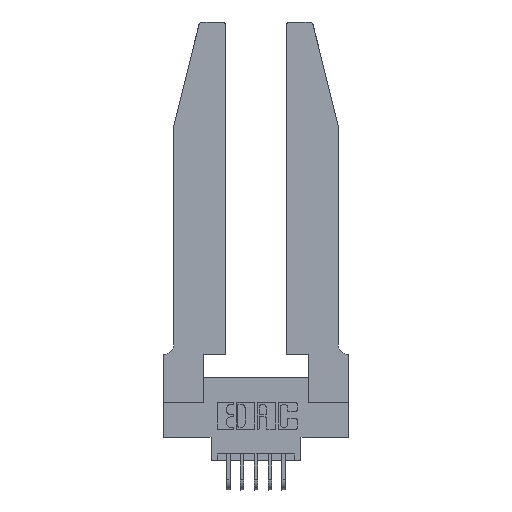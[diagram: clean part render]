
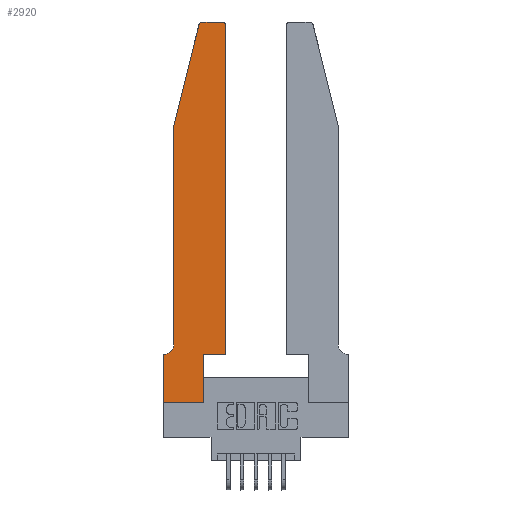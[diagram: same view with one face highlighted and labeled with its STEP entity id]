
A CAD part, top view. The second image highlights one B-rep face of the part: STEP entity #2920.
In plain terms, the highlighted planar face has unit normal (0, 0, 1).
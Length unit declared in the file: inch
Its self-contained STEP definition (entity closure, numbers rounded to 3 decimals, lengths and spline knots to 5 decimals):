
#267 = DIRECTION ( 'NONE',  ( 0., -1., 0. ) ) ;
#280 = EDGE_CURVE ( 'NONE', #4974, #8534, #6755, .T. ) ;
#390 = LINE ( 'NONE', #2423, #12693 ) ;
#575 = CARTESIAN_POINT ( 'NONE',  ( 0.4205, 2.72, 0.37 ) ) ;
#576 = DIRECTION ( 'NONE',  ( 1., 0., 0. ) ) ;
#625 = DIRECTION ( 'NONE',  ( 1., 0., 0. ) ) ;
#717 = VECTOR ( 'NONE', #1704, 39.37008 ) ;
#777 = DIRECTION ( 'NONE',  ( 1., 0., 0. ) ) ;
#1067 = ORIENTED_EDGE ( 'NONE', *, *, #4569, .T. ) ;
#1070 = VERTEX_POINT ( 'NONE', #10532 ) ;
#1077 = EDGE_CURVE ( 'NONE', #4889, #1070, #390, .T. ) ;
#1092 = VECTOR ( 'NONE', #5197, 39.37008 ) ;
#1368 = VECTOR ( 'NONE', #12959, 39.37008 ) ;
#1704 = DIRECTION ( 'NONE',  ( 0., 1., 0. ) ) ;
#1723 = CARTESIAN_POINT ( 'NONE',  ( 0.2865, 0.35, 0.37 ) ) ;
#1918 = DIRECTION ( 'NONE',  ( 0., 0., 1. ) ) ;
#2266 = CARTESIAN_POINT ( 'NONE',  ( 0.4505, 0.35, 0.37 ) ) ;
#2324 = ORIENTED_EDGE ( 'NONE', *, *, #12569, .T. ) ;
#2423 = CARTESIAN_POINT ( 'NONE',  ( 0.0755, 2., 0.37 ) ) ;
#2869 = CARTESIAN_POINT ( 'NONE',  ( 0.2865, 0.35, 0.37 ) ) ;
#2920 = ADVANCED_FACE ( 'NONE', ( #13415 ), #8913, .T. ) ;
#2939 = CARTESIAN_POINT ( 'NONE',  ( 0., 0.35, 0.37 ) ) ;
#2942 = VERTEX_POINT ( 'NONE', #2939 ) ;
#2949 = VERTEX_POINT ( 'NONE', #1723 ) ;
#3039 = DIRECTION ( 'NONE',  ( -1., 0., 0. ) ) ;
#3297 = CARTESIAN_POINT ( 'NONE',  ( 0.284, 2.72, 0.37 ) ) ;
#3588 = VERTEX_POINT ( 'NONE', #6437 ) ;
#3754 = LINE ( 'NONE', #11415, #14758 ) ;
#3841 = EDGE_LOOP ( 'NONE', ( #4428, #14065, #12921, #6975, #9036, #13709, #1067, #14324, #2324, #7661, #10446, #6878 ) ) ;
#4404 = LINE ( 'NONE', #13679, #4600 ) ;
#4428 = ORIENTED_EDGE ( 'NONE', *, *, #12655, .T. ) ;
#4569 = EDGE_CURVE ( 'NONE', #2942, #5217, #13560, .T. ) ;
#4600 = VECTOR ( 'NONE', #576, 39.37008 ) ;
#4889 = VERTEX_POINT ( 'NONE', #7549 ) ;
#4959 = DIRECTION ( 'NONE',  ( -0.239, -0.971, 0. ) ) ;
#4974 = VERTEX_POINT ( 'NONE', #13524 ) ;
#5197 = DIRECTION ( 'NONE',  ( 0., 1., 0. ) ) ;
#5217 = VERTEX_POINT ( 'NONE', #7340 ) ;
#5251 = CARTESIAN_POINT ( 'NONE',  ( 0.2865, 0., 0.37 ) ) ;
#5362 = CARTESIAN_POINT ( 'NONE',  ( 0.0055, 0.42, 0.37 ) ) ;
#5468 = DIRECTION ( 'NONE',  ( 0., 0., -1. ) ) ;
#5637 = CARTESIAN_POINT ( 'NONE',  ( 0.4505, 0.35, 0.37 ) ) ;
#5806 = DIRECTION ( 'NONE',  ( 0., -1., 0. ) ) ;
#5923 = EDGE_CURVE ( 'NONE', #2949, #13540, #8840, .T. ) ;
#6043 = CIRCLE ( 'NONE', #10051, 0.07 ) ;
#6257 = CARTESIAN_POINT ( 'NONE',  ( 0.0755, 2., 0.37 ) ) ;
#6437 = CARTESIAN_POINT ( 'NONE',  ( 0.4505, 2.72, 0.37 ) ) ;
#6447 = DIRECTION ( 'NONE',  ( -1., 0., 0. ) ) ;
#6755 = CIRCLE ( 'NONE', #14008, 0.03 ) ;
#6868 = LINE ( 'NONE', #11218, #1092 ) ;
#6878 = ORIENTED_EDGE ( 'NONE', *, *, #10476, .T. ) ;
#6975 = ORIENTED_EDGE ( 'NONE', *, *, #1077, .T. ) ;
#7340 = CARTESIAN_POINT ( 'NONE',  ( 0., 0., 0.37 ) ) ;
#7549 = CARTESIAN_POINT ( 'NONE',  ( 0.0755, 2., 0.37 ) ) ;
#7602 = VECTOR ( 'NONE', #267, 39.37008 ) ;
#7613 = EDGE_CURVE ( 'NONE', #11349, #2942, #8636, .T. ) ;
#7642 = CARTESIAN_POINT ( 'NONE',  ( 0., 0.35, 0.37 ) ) ;
#7661 = ORIENTED_EDGE ( 'NONE', *, *, #5923, .T. ) ;
#7710 = AXIS2_PLACEMENT_3D ( 'NONE', #575, #1918, #625 ) ;
#8254 = VECTOR ( 'NONE', #6447, 39.37008 ) ;
#8469 = AXIS2_PLACEMENT_3D ( 'NONE', #7642, #14876, #8807 ) ;
#8534 = VERTEX_POINT ( 'NONE', #14683 ) ;
#8636 = LINE ( 'NONE', #13449, #8254 ) ;
#8807 = DIRECTION ( 'NONE',  ( 1., 0., 0. ) ) ;
#8840 = LINE ( 'NONE', #5637, #1368 ) ;
#8913 = PLANE ( 'NONE',  #8469 ) ;
#9036 = ORIENTED_EDGE ( 'NONE', *, *, #12099, .T. ) ;
#9231 = EDGE_CURVE ( 'NONE', #13540, #3588, #6868, .T. ) ;
#9972 = VERTEX_POINT ( 'NONE', #10238 ) ;
#10051 = AXIS2_PLACEMENT_3D ( 'NONE', #5362, #5468, #3039 ) ;
#10238 = CARTESIAN_POINT ( 'NONE',  ( 0.4205, 2.75, 0.37 ) ) ;
#10446 = ORIENTED_EDGE ( 'NONE', *, *, #9231, .T. ) ;
#10476 = EDGE_CURVE ( 'NONE', #3588, #9972, #11497, .T. ) ;
#10532 = CARTESIAN_POINT ( 'NONE',  ( 0.0755, 0.42, 0.37 ) ) ;
#10546 = EDGE_CURVE ( 'NONE', #5217, #15064, #4404, .T. ) ;
#11218 = CARTESIAN_POINT ( 'NONE',  ( 0.4505, 0.35, 0.37 ) ) ;
#11280 = LINE ( 'NONE', #6257, #12208 ) ;
#11349 = VERTEX_POINT ( 'NONE', #13901 ) ;
#11415 = CARTESIAN_POINT ( 'NONE',  ( 0.2605, 2.75, 0.37 ) ) ;
#11465 = DIRECTION ( 'NONE',  ( -1., 0., 0. ) ) ;
#11497 = CIRCLE ( 'NONE', #7710, 0.03 ) ;
#11973 = EDGE_CURVE ( 'NONE', #8534, #4889, #11280, .T. ) ;
#12099 = EDGE_CURVE ( 'NONE', #1070, #11349, #6043, .T. ) ;
#12155 = CARTESIAN_POINT ( 'NONE',  ( 0., 0., 0.37 ) ) ;
#12208 = VECTOR ( 'NONE', #4959, 39.37008 ) ;
#12569 = EDGE_CURVE ( 'NONE', #15064, #2949, #15459, .T. ) ;
#12655 = EDGE_CURVE ( 'NONE', #9972, #4974, #3754, .T. ) ;
#12693 = VECTOR ( 'NONE', #5806, 39.37008 ) ;
#12921 = ORIENTED_EDGE ( 'NONE', *, *, #11973, .T. ) ;
#12959 = DIRECTION ( 'NONE',  ( 1., 0., 0. ) ) ;
#13415 = FACE_OUTER_BOUND ( 'NONE', #3841, .T. ) ;
#13449 = CARTESIAN_POINT ( 'NONE',  ( 0.0755, 0.35, 0.37 ) ) ;
#13524 = CARTESIAN_POINT ( 'NONE',  ( 0.284, 2.75, 0.37 ) ) ;
#13540 = VERTEX_POINT ( 'NONE', #2266 ) ;
#13560 = LINE ( 'NONE', #12155, #7602 ) ;
#13679 = CARTESIAN_POINT ( 'NONE',  ( 0., 0., 0.37 ) ) ;
#13709 = ORIENTED_EDGE ( 'NONE', *, *, #7613, .T. ) ;
#13901 = CARTESIAN_POINT ( 'NONE',  ( 0.0055, 0.35, 0.37 ) ) ;
#14008 = AXIS2_PLACEMENT_3D ( 'NONE', #3297, #15134, #777 ) ;
#14065 = ORIENTED_EDGE ( 'NONE', *, *, #280, .T. ) ;
#14324 = ORIENTED_EDGE ( 'NONE', *, *, #10546, .T. ) ;
#14683 = CARTESIAN_POINT ( 'NONE',  ( 0.25487, 2.72718, 0.37 ) ) ;
#14758 = VECTOR ( 'NONE', #11465, 39.37008 ) ;
#14876 = DIRECTION ( 'NONE',  ( 0., 0., 1. ) ) ;
#15064 = VERTEX_POINT ( 'NONE', #5251 ) ;
#15134 = DIRECTION ( 'NONE',  ( 0., 0., 1. ) ) ;
#15459 = LINE ( 'NONE', #2869, #717 ) ;
